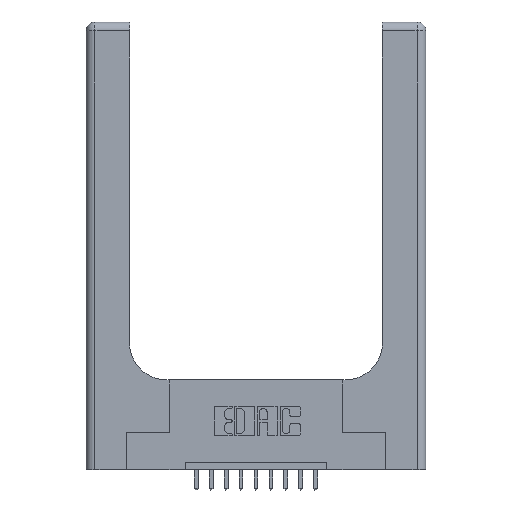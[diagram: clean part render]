
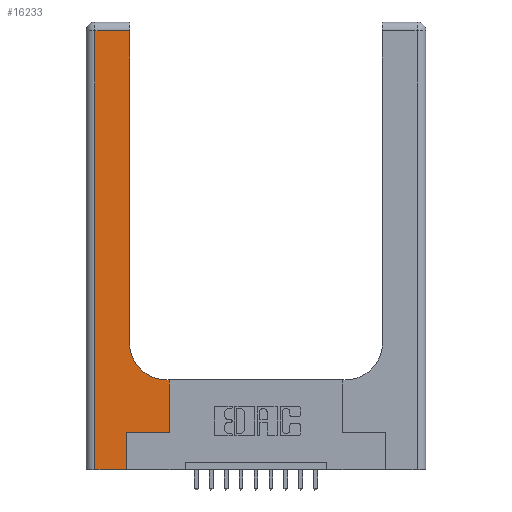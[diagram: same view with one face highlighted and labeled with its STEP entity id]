
A CAD part, top view. The second image highlights one B-rep face of the part: STEP entity #16233.
In plain terms, the highlighted planar face has unit normal (0, 0, 1).
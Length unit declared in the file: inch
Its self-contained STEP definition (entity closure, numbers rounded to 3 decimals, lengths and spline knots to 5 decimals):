
#172 = CARTESIAN_POINT ( 'NONE',  ( 0.5585, 0.25, 0.37 ) ) ;
#745 = VERTEX_POINT ( 'NONE', #11309 ) ;
#940 = AXIS2_PLACEMENT_3D ( 'NONE', #8712, #16348, #16138 ) ;
#953 = CARTESIAN_POINT ( 'NONE',  ( 0.2915, 0.6, 0.37 ) ) ;
#1081 = EDGE_CURVE ( 'NONE', #8054, #14873, #5200, .T. ) ;
#1126 = VECTOR ( 'NONE', #13873, 39.37008 ) ;
#1251 = VECTOR ( 'NONE', #16222, 39.37008 ) ;
#1665 = EDGE_CURVE ( 'NONE', #4559, #12581, #6788, .T. ) ;
#1790 = EDGE_CURVE ( 'NONE', #8565, #12971, #12553, .T. ) ;
#2724 = CARTESIAN_POINT ( 'NONE',  ( 0.269, 0., 0.37 ) ) ;
#2757 = CARTESIAN_POINT ( 'NONE',  ( 0.2915, 2.94, 0.37 ) ) ;
#3821 = CARTESIAN_POINT ( 'NONE',  ( 0.06, 0., 0.37 ) ) ;
#3996 = VECTOR ( 'NONE', #6364, 39.37008 ) ;
#4063 = EDGE_CURVE ( 'NONE', #12581, #8565, #11756, .T. ) ;
#4315 = CARTESIAN_POINT ( 'NONE',  ( 0.269, 0., 0.37 ) ) ;
#4559 = VERTEX_POINT ( 'NONE', #5415 ) ;
#4694 = ORIENTED_EDGE ( 'NONE', *, *, #4063, .T. ) ;
#4897 = CARTESIAN_POINT ( 'NONE',  ( 0., 2.94, 0.37 ) ) ;
#4994 = VECTOR ( 'NONE', #8660, 39.37008 ) ;
#5162 = VECTOR ( 'NONE', #7685, 39.37008 ) ;
#5200 = LINE ( 'NONE', #5899, #1251 ) ;
#5293 = CARTESIAN_POINT ( 'NONE',  ( 0.5585, 0.25, 0.37 ) ) ;
#5415 = CARTESIAN_POINT ( 'NONE',  ( 0.5585, 0.6, 0.37 ) ) ;
#5521 = CARTESIAN_POINT ( 'NONE',  ( 0.2915, 0.85, 0.37 ) ) ;
#5528 = VECTOR ( 'NONE', #16431, 39.37008 ) ;
#5647 = EDGE_LOOP ( 'NONE', ( #10742, #13898, #11882, #15672, #13699, #14972, #6446, #15194, #4694 ) ) ;
#5899 = CARTESIAN_POINT ( 'NONE',  ( 0.269, 0.25, 0.37 ) ) ;
#6364 = DIRECTION ( 'NONE',  ( 0., 1., 0. ) ) ;
#6417 = EDGE_CURVE ( 'NONE', #12971, #745, #16108, .T. ) ;
#6446 = ORIENTED_EDGE ( 'NONE', *, *, #15391, .T. ) ;
#6672 = LINE ( 'NONE', #15142, #1126 ) ;
#6788 = LINE ( 'NONE', #953, #4994 ) ;
#7205 = PLANE ( 'NONE',  #940 ) ;
#7349 = AXIS2_PLACEMENT_3D ( 'NONE', #15538, #11624, #14327 ) ;
#7685 = DIRECTION ( 'NONE',  ( 0., 1., 0. ) ) ;
#7871 = VERTEX_POINT ( 'NONE', #2724 ) ;
#7901 = EDGE_CURVE ( 'NONE', #7871, #8054, #15252, .T. ) ;
#8054 = VERTEX_POINT ( 'NONE', #13824 ) ;
#8565 = VERTEX_POINT ( 'NONE', #5521 ) ;
#8660 = DIRECTION ( 'NONE',  ( -1., 0., 0. ) ) ;
#8712 = CARTESIAN_POINT ( 'NONE',  ( 0., 3., 0.37 ) ) ;
#9299 = VERTEX_POINT ( 'NONE', #3821 ) ;
#9509 = CARTESIAN_POINT ( 'NONE',  ( 0.06, 3., 0.37 ) ) ;
#10195 = CARTESIAN_POINT ( 'NONE',  ( 0.2915, 3., 0.37 ) ) ;
#10642 = VECTOR ( 'NONE', #15627, 39.37008 ) ;
#10742 = ORIENTED_EDGE ( 'NONE', *, *, #1790, .T. ) ;
#11085 = EDGE_CURVE ( 'NONE', #9299, #7871, #6672, .T. ) ;
#11309 = CARTESIAN_POINT ( 'NONE',  ( 0.06, 2.94, 0.37 ) ) ;
#11624 = DIRECTION ( 'NONE',  ( 0., 0., -1. ) ) ;
#11756 = CIRCLE ( 'NONE', #7349, 0.25 ) ;
#11802 = VECTOR ( 'NONE', #12196, 39.37008 ) ;
#11882 = ORIENTED_EDGE ( 'NONE', *, *, #13171, .T. ) ;
#12161 = LINE ( 'NONE', #172, #5162 ) ;
#12196 = DIRECTION ( 'NONE',  ( 0., -1., 0. ) ) ;
#12553 = LINE ( 'NONE', #10195, #3996 ) ;
#12581 = VERTEX_POINT ( 'NONE', #16029 ) ;
#12971 = VERTEX_POINT ( 'NONE', #2757 ) ;
#13171 = EDGE_CURVE ( 'NONE', #745, #9299, #14429, .T. ) ;
#13699 = ORIENTED_EDGE ( 'NONE', *, *, #7901, .T. ) ;
#13824 = CARTESIAN_POINT ( 'NONE',  ( 0.269, 0.25, 0.37 ) ) ;
#13873 = DIRECTION ( 'NONE',  ( 1., 0., 0. ) ) ;
#13898 = ORIENTED_EDGE ( 'NONE', *, *, #6417, .T. ) ;
#14327 = DIRECTION ( 'NONE',  ( 1., 0., 0. ) ) ;
#14429 = LINE ( 'NONE', #9509, #11802 ) ;
#14873 = VERTEX_POINT ( 'NONE', #5293 ) ;
#14972 = ORIENTED_EDGE ( 'NONE', *, *, #1081, .T. ) ;
#15142 = CARTESIAN_POINT ( 'NONE',  ( 0., 0., 0.37 ) ) ;
#15194 = ORIENTED_EDGE ( 'NONE', *, *, #1665, .T. ) ;
#15252 = LINE ( 'NONE', #4315, #10642 ) ;
#15310 = FACE_OUTER_BOUND ( 'NONE', #5647, .T. ) ;
#15391 = EDGE_CURVE ( 'NONE', #14873, #4559, #12161, .T. ) ;
#15538 = CARTESIAN_POINT ( 'NONE',  ( 0.5415, 0.85, 0.37 ) ) ;
#15627 = DIRECTION ( 'NONE',  ( 0., 1., 0. ) ) ;
#15672 = ORIENTED_EDGE ( 'NONE', *, *, #11085, .T. ) ;
#16029 = CARTESIAN_POINT ( 'NONE',  ( 0.5415, 0.6, 0.37 ) ) ;
#16108 = LINE ( 'NONE', #4897, #5528 ) ;
#16138 = DIRECTION ( 'NONE',  ( -1., 0., 0. ) ) ;
#16222 = DIRECTION ( 'NONE',  ( 1., 0., 0. ) ) ;
#16233 = ADVANCED_FACE ( 'NONE', ( #15310 ), #7205, .F. ) ;
#16348 = DIRECTION ( 'NONE',  ( 0., 0., -1. ) ) ;
#16431 = DIRECTION ( 'NONE',  ( -1., 0., 0. ) ) ;
